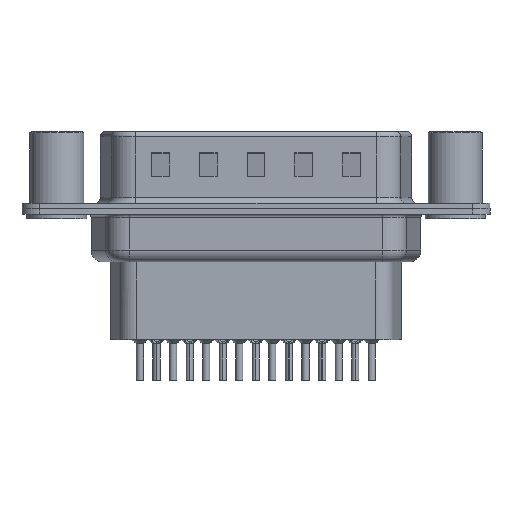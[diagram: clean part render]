
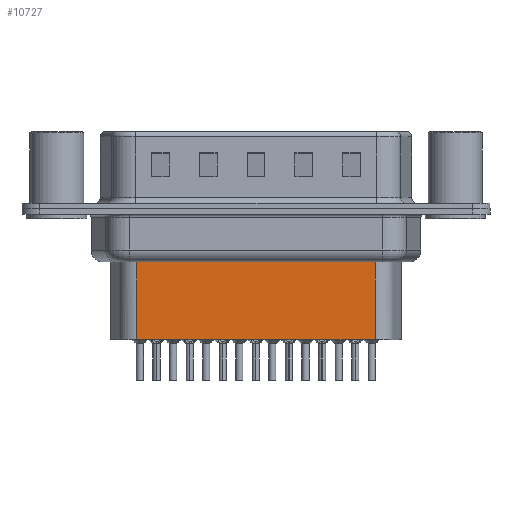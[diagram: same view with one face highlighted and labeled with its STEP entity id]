
A CAD part, front view. The second image highlights one B-rep face of the part: STEP entity #10727.
In plain terms, the highlighted planar face has unit normal (0, -1, 0).
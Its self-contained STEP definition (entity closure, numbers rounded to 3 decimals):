
#174 = VECTOR ( 'NONE', #6860, 1000. ) ;
#179 = ORIENTED_EDGE ( 'NONE', *, *, #8264, .T. ) ;
#723 = ORIENTED_EDGE ( 'NONE', *, *, #13368, .F. ) ;
#2395 = AXIS2_PLACEMENT_3D ( 'NONE', #20809, #3319, #5014 ) ;
#3319 = DIRECTION ( 'NONE',  ( 0., -1., 0. ) ) ;
#3548 = VECTOR ( 'NONE', #11929, 1000. ) ;
#3719 = ORIENTED_EDGE ( 'NONE', *, *, #13096, .T. ) ;
#5014 = DIRECTION ( 'NONE',  ( 1., 0., 0. ) ) ;
#5553 = CARTESIAN_POINT ( 'NONE',  ( 6.681, -3.5, -3.1 ) ) ;
#5904 = EDGE_LOOP ( 'NONE', ( #723, #179, #3719, #17042 ) ) ;
#6860 = DIRECTION ( 'NONE',  ( -1., 0., 0. ) ) ;
#6867 = CARTESIAN_POINT ( 'NONE',  ( 26.619, -3.5, -3.1 ) ) ;
#8264 = EDGE_CURVE ( 'NONE', #13686, #14209, #8644, .T. ) ;
#8511 = LINE ( 'NONE', #10001, #9245 ) ;
#8644 = LINE ( 'NONE', #21003, #174 ) ;
#9048 = VERTEX_POINT ( 'NONE', #12090 ) ;
#9245 = VECTOR ( 'NONE', #10315, 1000. ) ;
#9662 = VECTOR ( 'NONE', #12393, 1000. ) ;
#10001 = CARTESIAN_POINT ( 'NONE',  ( 6.681, -3.5, -10.95 ) ) ;
#10315 = DIRECTION ( 'NONE',  ( -1., 0., 0. ) ) ;
#10727 = ADVANCED_FACE ( 'NONE', ( #16998 ), #17328, .T. ) ;
#11627 = EDGE_CURVE ( 'NONE', #9048, #15793, #8511, .T. ) ;
#11929 = DIRECTION ( 'NONE',  ( 0., 0., -1. ) ) ;
#12090 = CARTESIAN_POINT ( 'NONE',  ( 26.619, -3.5, -10.95 ) ) ;
#12393 = DIRECTION ( 'NONE',  ( 0., 0., -1. ) ) ;
#13096 = EDGE_CURVE ( 'NONE', #14209, #15793, #15865, .T. ) ;
#13368 = EDGE_CURVE ( 'NONE', #13686, #9048, #15095, .T. ) ;
#13686 = VERTEX_POINT ( 'NONE', #18356 ) ;
#14209 = VERTEX_POINT ( 'NONE', #18407 ) ;
#15095 = LINE ( 'NONE', #6867, #3548 ) ;
#15793 = VERTEX_POINT ( 'NONE', #18607 ) ;
#15865 = LINE ( 'NONE', #5553, #9662 ) ;
#16998 = FACE_OUTER_BOUND ( 'NONE', #5904, .T. ) ;
#17042 = ORIENTED_EDGE ( 'NONE', *, *, #11627, .F. ) ;
#17328 = PLANE ( 'NONE',  #2395 ) ;
#18356 = CARTESIAN_POINT ( 'NONE',  ( 26.619, -3.5, -4.097 ) ) ;
#18407 = CARTESIAN_POINT ( 'NONE',  ( 6.681, -3.5, -4.097 ) ) ;
#18607 = CARTESIAN_POINT ( 'NONE',  ( 6.681, -3.5, -10.95 ) ) ;
#20809 = CARTESIAN_POINT ( 'NONE',  ( 6.681, -3.5, -3.1 ) ) ;
#21003 = CARTESIAN_POINT ( 'NONE',  ( 6.434, -3.5, -4.097 ) ) ;
